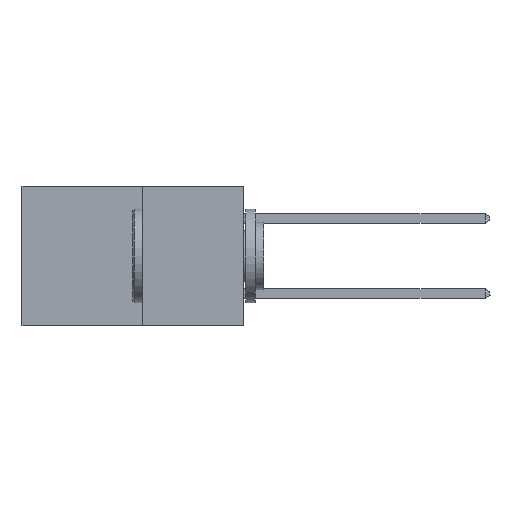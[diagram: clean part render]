
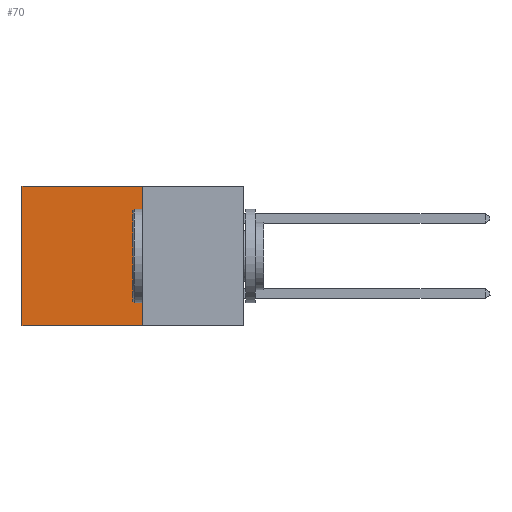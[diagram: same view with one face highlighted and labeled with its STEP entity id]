
A CAD part, left-side view. The second image highlights one B-rep face of the part: STEP entity #70.
In plain terms, the highlighted planar face has unit normal (-1, 0, 0).
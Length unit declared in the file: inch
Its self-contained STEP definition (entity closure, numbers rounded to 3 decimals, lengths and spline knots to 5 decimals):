
#70 = ADVANCED_FACE ( 'NONE', ( #8865 ), #5833, .F. ) ;
#222 = DIRECTION ( 'NONE',  ( 1., 0., 0. ) ) ;
#275 = DIRECTION ( 'NONE',  ( 0., 0., -1. ) ) ;
#564 = EDGE_CURVE ( 'NONE', #7236, #6994, #2206, .T. ) ;
#1159 = EDGE_CURVE ( 'NONE', #4794, #8394, #3925, .T. ) ;
#1999 = CARTESIAN_POINT ( 'NONE',  ( 0.277, 0.27, -0.37 ) ) ;
#2040 = CARTESIAN_POINT ( 'NONE',  ( 0.277, 0.59, -0.37 ) ) ;
#2069 = CARTESIAN_POINT ( 'NONE',  ( 0.277, 0.27, -0.37 ) ) ;
#2206 = LINE ( 'NONE', #3155, #8751 ) ;
#2223 = CARTESIAN_POINT ( 'NONE',  ( 0.277, 0.59, 0. ) ) ;
#2296 = VECTOR ( 'NONE', #6073, 39.37008 ) ;
#2675 = CARTESIAN_POINT ( 'NONE',  ( 0.277, 0.59, -0.37 ) ) ;
#3155 = CARTESIAN_POINT ( 'NONE',  ( 0.277, 0.27, 0. ) ) ;
#3841 = LINE ( 'NONE', #2040, #8171 ) ;
#3925 = LINE ( 'NONE', #7482, #10899 ) ;
#4785 = DIRECTION ( 'NONE',  ( 0., 1., 0. ) ) ;
#4794 = VERTEX_POINT ( 'NONE', #2069 ) ;
#5457 = ORIENTED_EDGE ( 'NONE', *, *, #9247, .T. ) ;
#5469 = ORIENTED_EDGE ( 'NONE', *, *, #1159, .F. ) ;
#5644 = ORIENTED_EDGE ( 'NONE', *, *, #6818, .F. ) ;
#5779 = ORIENTED_EDGE ( 'NONE', *, *, #564, .T. ) ;
#5833 = PLANE ( 'NONE',  #6142 ) ;
#6073 = DIRECTION ( 'NONE',  ( 0., 0., -1. ) ) ;
#6142 = AXIS2_PLACEMENT_3D ( 'NONE', #1999, #222, #10946 ) ;
#6149 = CARTESIAN_POINT ( 'NONE',  ( 0.277, 0.27, -0.37 ) ) ;
#6373 = DIRECTION ( 'NONE',  ( 0., 1., 0. ) ) ;
#6818 = EDGE_CURVE ( 'NONE', #7236, #4794, #6847, .T. ) ;
#6847 = LINE ( 'NONE', #6149, #2296 ) ;
#6994 = VERTEX_POINT ( 'NONE', #2223 ) ;
#7236 = VERTEX_POINT ( 'NONE', #10167 ) ;
#7482 = CARTESIAN_POINT ( 'NONE',  ( 0.277, 0.27, -0.37 ) ) ;
#8171 = VECTOR ( 'NONE', #275, 39.37008 ) ;
#8394 = VERTEX_POINT ( 'NONE', #2675 ) ;
#8751 = VECTOR ( 'NONE', #6373, 39.37008 ) ;
#8865 = FACE_OUTER_BOUND ( 'NONE', #9832, .T. ) ;
#9247 = EDGE_CURVE ( 'NONE', #6994, #8394, #3841, .T. ) ;
#9832 = EDGE_LOOP ( 'NONE', ( #5457, #5469, #5644, #5779 ) ) ;
#10167 = CARTESIAN_POINT ( 'NONE',  ( 0.277, 0.27, 0. ) ) ;
#10899 = VECTOR ( 'NONE', #4785, 39.37008 ) ;
#10946 = DIRECTION ( 'NONE',  ( 0., 0., -1. ) ) ;
